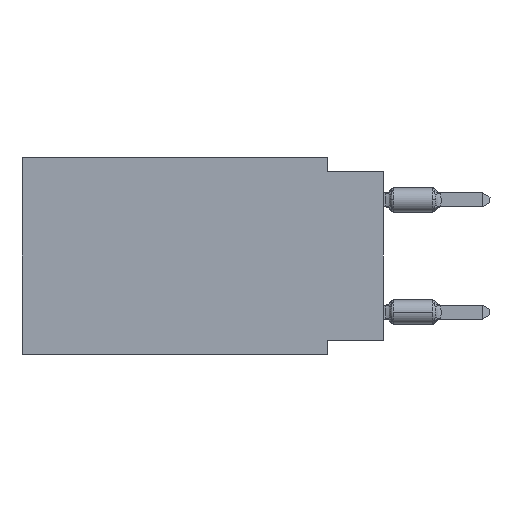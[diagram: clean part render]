
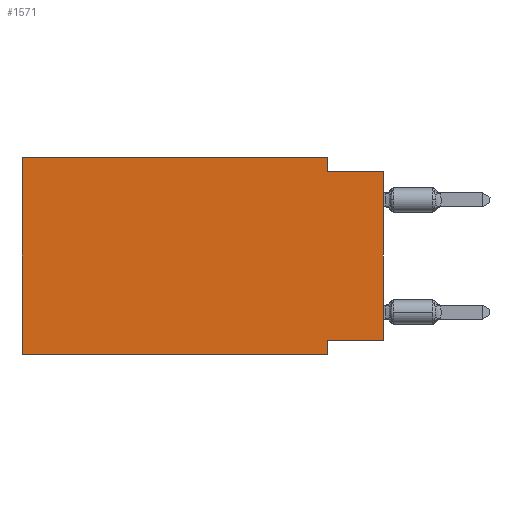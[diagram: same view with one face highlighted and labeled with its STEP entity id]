
A CAD part, left-side view. The second image highlights one B-rep face of the part: STEP entity #1571.
In plain terms, the highlighted planar face has unit normal (-1, 0, 0).
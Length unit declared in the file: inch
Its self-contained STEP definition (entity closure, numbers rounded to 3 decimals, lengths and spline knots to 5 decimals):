
#61 = DIRECTION ( 'NONE',  ( 1., 0., 0. ) ) ;
#897 = VECTOR ( 'NONE', #9505, 39.37008 ) ;
#1145 = ORIENTED_EDGE ( 'NONE', *, *, #6824, .F. ) ;
#1273 = DIRECTION ( 'NONE',  ( 0., 0., -1. ) ) ;
#1529 = CARTESIAN_POINT ( 'NONE',  ( 0., 0.645, 0. ) ) ;
#1571 = ADVANCED_FACE ( 'NONE', ( #20203 ), #2289, .F. ) ;
#1651 = VERTEX_POINT ( 'NONE', #15067 ) ;
#2289 = PLANE ( 'NONE',  #11883 ) ;
#2644 = VECTOR ( 'NONE', #18018, 39.37008 ) ;
#2689 = VECTOR ( 'NONE', #1273, 39.37008 ) ;
#3131 = EDGE_CURVE ( 'NONE', #24003, #12151, #9391, .T. ) ;
#3632 = DIRECTION ( 'NONE',  ( 0., -1., 0. ) ) ;
#4225 = DIRECTION ( 'NONE',  ( 0., 1., 0. ) ) ;
#4367 = CARTESIAN_POINT ( 'NONE',  ( 0., 0.1, -0.025 ) ) ;
#5451 = EDGE_CURVE ( 'NONE', #1651, #12151, #24523, .T. ) ;
#5673 = ORIENTED_EDGE ( 'NONE', *, *, #17384, .F. ) ;
#5839 = LINE ( 'NONE', #1529, #897 ) ;
#6619 = CARTESIAN_POINT ( 'NONE',  ( 0., 0.645, -0.35 ) ) ;
#6765 = VECTOR ( 'NONE', #10712, 39.37008 ) ;
#6824 = EDGE_CURVE ( 'NONE', #11017, #14477, #25606, .T. ) ;
#7043 = CARTESIAN_POINT ( 'NONE',  ( 0., 0.1, -0.35 ) ) ;
#7427 = CARTESIAN_POINT ( 'NONE',  ( 0., 0., -0.025 ) ) ;
#7659 = VERTEX_POINT ( 'NONE', #19617 ) ;
#8979 = VECTOR ( 'NONE', #3632, 39.37008 ) ;
#9391 = LINE ( 'NONE', #7043, #2689 ) ;
#9505 = DIRECTION ( 'NONE',  ( 0., 0., 1. ) ) ;
#10712 = DIRECTION ( 'NONE',  ( 0., -1., 0. ) ) ;
#10967 = VECTOR ( 'NONE', #19936, 39.37008 ) ;
#11017 = VERTEX_POINT ( 'NONE', #4367 ) ;
#11086 = EDGE_CURVE ( 'NONE', #7659, #24003, #15990, .T. ) ;
#11225 = CARTESIAN_POINT ( 'NONE',  ( 0., 0.645, 0. ) ) ;
#11244 = CARTESIAN_POINT ( 'NONE',  ( 0., 0., -0.025 ) ) ;
#11689 = LINE ( 'NONE', #22025, #10967 ) ;
#11883 = AXIS2_PLACEMENT_3D ( 'NONE', #12091, #61, #20066 ) ;
#12091 = CARTESIAN_POINT ( 'NONE',  ( 0., 0.645, 0. ) ) ;
#12151 = VERTEX_POINT ( 'NONE', #17922 ) ;
#12433 = ORIENTED_EDGE ( 'NONE', *, *, #15018, .F. ) ;
#12439 = CARTESIAN_POINT ( 'NONE',  ( 0., 0.1, -0.325 ) ) ;
#14477 = VERTEX_POINT ( 'NONE', #11244 ) ;
#14577 = DIRECTION ( 'NONE',  ( 0., -1., 0. ) ) ;
#15018 = EDGE_CURVE ( 'NONE', #1651, #19436, #5839, .T. ) ;
#15067 = CARTESIAN_POINT ( 'NONE',  ( 0., 0.645, -0.35 ) ) ;
#15310 = CARTESIAN_POINT ( 'NONE',  ( 0., 0.645, 0. ) ) ;
#15990 = LINE ( 'NONE', #16124, #17826 ) ;
#16124 = CARTESIAN_POINT ( 'NONE',  ( 0., 0., -0.325 ) ) ;
#16418 = EDGE_CURVE ( 'NONE', #7659, #14477, #11689, .T. ) ;
#16462 = LINE ( 'NONE', #24441, #2644 ) ;
#17384 = EDGE_CURVE ( 'NONE', #21065, #11017, #16462, .T. ) ;
#17432 = VECTOR ( 'NONE', #14577, 39.37008 ) ;
#17826 = VECTOR ( 'NONE', #4225, 39.37008 ) ;
#17922 = CARTESIAN_POINT ( 'NONE',  ( 0., 0.1, -0.35 ) ) ;
#18018 = DIRECTION ( 'NONE',  ( 0., 0., -1. ) ) ;
#18962 = CARTESIAN_POINT ( 'NONE',  ( 0., 0.1, 0. ) ) ;
#19436 = VERTEX_POINT ( 'NONE', #15310 ) ;
#19617 = CARTESIAN_POINT ( 'NONE',  ( 0., 0., -0.325 ) ) ;
#19891 = EDGE_CURVE ( 'NONE', #19436, #21065, #21299, .T. ) ;
#19936 = DIRECTION ( 'NONE',  ( 0., 0., 1. ) ) ;
#20066 = DIRECTION ( 'NONE',  ( 0., 0., -1. ) ) ;
#20203 = FACE_OUTER_BOUND ( 'NONE', #20471, .T. ) ;
#20471 = EDGE_LOOP ( 'NONE', ( #24628, #1145, #5673, #21909, #12433, #21635, #24553, #24221 ) ) ;
#21065 = VERTEX_POINT ( 'NONE', #18962 ) ;
#21299 = LINE ( 'NONE', #11225, #6765 ) ;
#21635 = ORIENTED_EDGE ( 'NONE', *, *, #5451, .T. ) ;
#21909 = ORIENTED_EDGE ( 'NONE', *, *, #19891, .F. ) ;
#22025 = CARTESIAN_POINT ( 'NONE',  ( 0., 0., 0. ) ) ;
#24003 = VERTEX_POINT ( 'NONE', #12439 ) ;
#24221 = ORIENTED_EDGE ( 'NONE', *, *, #11086, .F. ) ;
#24441 = CARTESIAN_POINT ( 'NONE',  ( 0., 0.1, 0. ) ) ;
#24523 = LINE ( 'NONE', #6619, #17432 ) ;
#24553 = ORIENTED_EDGE ( 'NONE', *, *, #3131, .F. ) ;
#24628 = ORIENTED_EDGE ( 'NONE', *, *, #16418, .T. ) ;
#25606 = LINE ( 'NONE', #7427, #8979 ) ;
